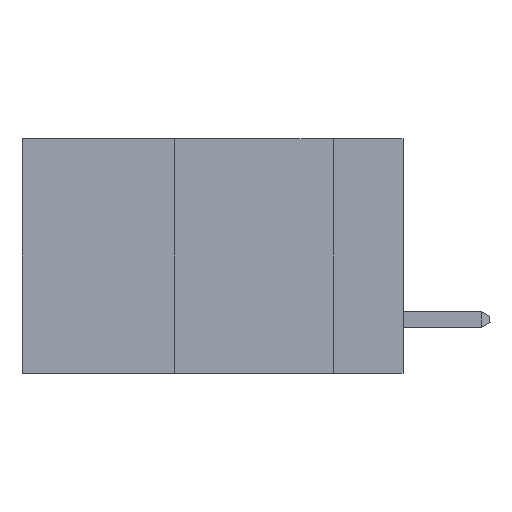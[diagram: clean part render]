
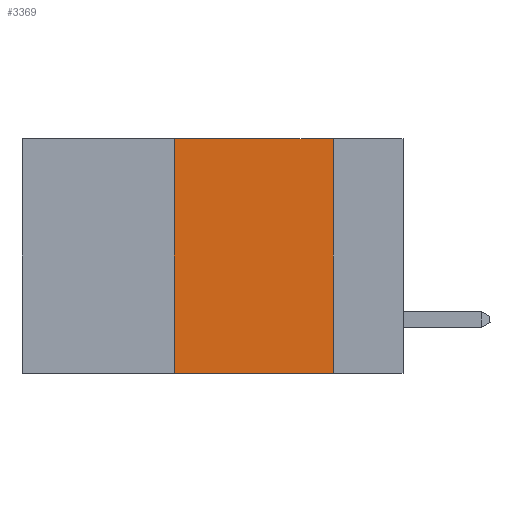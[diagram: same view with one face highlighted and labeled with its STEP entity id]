
A CAD part, left-side view. The second image highlights one B-rep face of the part: STEP entity #3369.
In plain terms, the highlighted planar face has unit normal (-1, 0, 0).
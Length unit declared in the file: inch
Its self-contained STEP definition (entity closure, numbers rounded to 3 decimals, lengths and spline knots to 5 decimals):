
#1163 = VECTOR ( 'NONE', #29226, 39.37008 ) ;
#2233 = ORIENTED_EDGE ( 'NONE', *, *, #30002, .T. ) ;
#2420 = VECTOR ( 'NONE', #24394, 39.37008 ) ;
#2488 = DIRECTION ( 'NONE',  ( 1., 0., 0. ) ) ;
#3369 = ADVANCED_FACE ( 'NONE', ( #16527 ), #32173, .F. ) ;
#3623 = ORIENTED_EDGE ( 'NONE', *, *, #13497, .F. ) ;
#8330 = VECTOR ( 'NONE', #24729, 39.37008 ) ;
#10050 = EDGE_CURVE ( 'NONE', #35663, #28814, #10442, .T. ) ;
#10442 = LINE ( 'NONE', #15502, #2420 ) ;
#13194 = VECTOR ( 'NONE', #16499, 39.37008 ) ;
#13497 = EDGE_CURVE ( 'NONE', #26752, #35663, #24966, .T. ) ;
#15502 = CARTESIAN_POINT ( 'NONE',  ( 0., 0.11, 0. ) ) ;
#16499 = DIRECTION ( 'NONE',  ( 0., 0., 1. ) ) ;
#16527 = FACE_OUTER_BOUND ( 'NONE', #25169, .T. ) ;
#17658 = ORIENTED_EDGE ( 'NONE', *, *, #10050, .F. ) ;
#19454 = LINE ( 'NONE', #31273, #13194 ) ;
#21772 = CARTESIAN_POINT ( 'NONE',  ( 0., 0.6, -0.37 ) ) ;
#21967 = CARTESIAN_POINT ( 'NONE',  ( 0., 0.11, 0. ) ) ;
#23334 = DIRECTION ( 'NONE',  ( 0., 0., -1. ) ) ;
#24168 = LINE ( 'NONE', #21772, #8330 ) ;
#24394 = DIRECTION ( 'NONE',  ( 0., 0., -1. ) ) ;
#24729 = DIRECTION ( 'NONE',  ( 0., -1., 0. ) ) ;
#24966 = LINE ( 'NONE', #26214, #1163 ) ;
#25169 = EDGE_LOOP ( 'NONE', ( #17658, #3623, #31132, #2233 ) ) ;
#26214 = CARTESIAN_POINT ( 'NONE',  ( 0., 0.6, 0. ) ) ;
#26752 = VERTEX_POINT ( 'NONE', #37499 ) ;
#28814 = VERTEX_POINT ( 'NONE', #36720 ) ;
#29226 = DIRECTION ( 'NONE',  ( 0., -1., 0. ) ) ;
#30002 = EDGE_CURVE ( 'NONE', #36567, #28814, #24168, .T. ) ;
#31132 = ORIENTED_EDGE ( 'NONE', *, *, #31416, .F. ) ;
#31273 = CARTESIAN_POINT ( 'NONE',  ( 0., 0.36, 0. ) ) ;
#31416 = EDGE_CURVE ( 'NONE', #36567, #26752, #19454, .T. ) ;
#32173 = PLANE ( 'NONE',  #35421 ) ;
#35110 = CARTESIAN_POINT ( 'NONE',  ( 0., 0.36, -0.37 ) ) ;
#35421 = AXIS2_PLACEMENT_3D ( 'NONE', #38069, #2488, #23334 ) ;
#35663 = VERTEX_POINT ( 'NONE', #21967 ) ;
#36567 = VERTEX_POINT ( 'NONE', #35110 ) ;
#36720 = CARTESIAN_POINT ( 'NONE',  ( 0., 0.11, -0.37 ) ) ;
#37499 = CARTESIAN_POINT ( 'NONE',  ( 0., 0.36, 0. ) ) ;
#38069 = CARTESIAN_POINT ( 'NONE',  ( 0., 0.6, 0. ) ) ;
